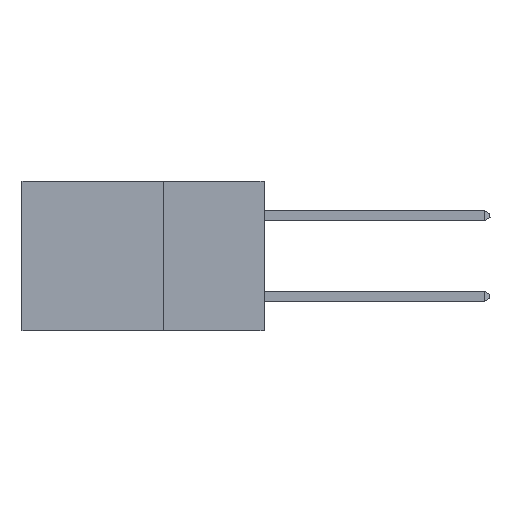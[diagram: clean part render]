
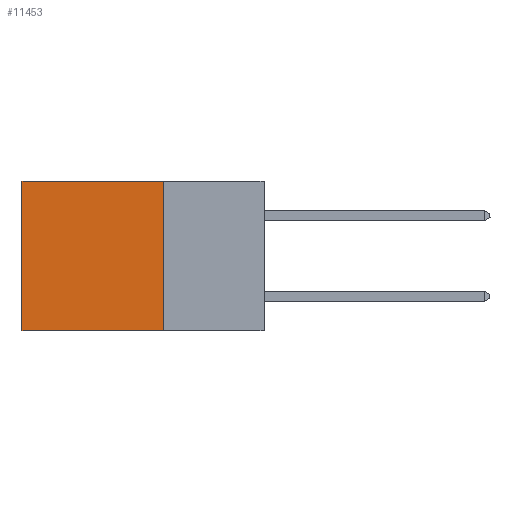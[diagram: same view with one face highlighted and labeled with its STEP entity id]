
A CAD part, left-side view. The second image highlights one B-rep face of the part: STEP entity #11453.
In plain terms, the highlighted planar face has unit normal (-1, 0, 0).
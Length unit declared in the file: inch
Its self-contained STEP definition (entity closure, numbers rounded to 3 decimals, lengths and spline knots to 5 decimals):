
#175 = AXIS2_PLACEMENT_3D ( 'NONE', #6943, #1509, #12089 ) ;
#1000 = ORIENTED_EDGE ( 'NONE', *, *, #13072, .F. ) ;
#1509 = DIRECTION ( 'NONE',  ( 1., 0., 0. ) ) ;
#1548 = EDGE_CURVE ( 'NONE', #6467, #7596, #8917, .T. ) ;
#3827 = CARTESIAN_POINT ( 'NONE',  ( 0.298, 0.6, -0.37 ) ) ;
#4586 = DIRECTION ( 'NONE',  ( 0., 0., -1. ) ) ;
#4882 = VECTOR ( 'NONE', #9130, 39.37008 ) ;
#6467 = VERTEX_POINT ( 'NONE', #10850 ) ;
#6473 = CARTESIAN_POINT ( 'NONE',  ( 0.298, 0.25, -0.37 ) ) ;
#6724 = LINE ( 'NONE', #9670, #13914 ) ;
#6943 = CARTESIAN_POINT ( 'NONE',  ( 0.298, 0.25, 0. ) ) ;
#7167 = VERTEX_POINT ( 'NONE', #3827 ) ;
#7596 = VERTEX_POINT ( 'NONE', #7931 ) ;
#7931 = CARTESIAN_POINT ( 'NONE',  ( 0.298, 0.6, 0. ) ) ;
#8087 = VECTOR ( 'NONE', #16560, 39.37008 ) ;
#8239 = PLANE ( 'NONE',  #175 ) ;
#8670 = DIRECTION ( 'NONE',  ( 0., 0., -1. ) ) ;
#8917 = LINE ( 'NONE', #13822, #8087 ) ;
#9020 = VERTEX_POINT ( 'NONE', #11935 ) ;
#9130 = DIRECTION ( 'NONE',  ( 0., 1., 0. ) ) ;
#9481 = LINE ( 'NONE', #15187, #11712 ) ;
#9642 = ORIENTED_EDGE ( 'NONE', *, *, #15500, .F. ) ;
#9670 = CARTESIAN_POINT ( 'NONE',  ( 0.298, 0.6, 0. ) ) ;
#9924 = FACE_OUTER_BOUND ( 'NONE', #10275, .T. ) ;
#10240 = ORIENTED_EDGE ( 'NONE', *, *, #1548, .T. ) ;
#10275 = EDGE_LOOP ( 'NONE', ( #15477, #9642, #1000, #10240 ) ) ;
#10850 = CARTESIAN_POINT ( 'NONE',  ( 0.298, 0.25, 0. ) ) ;
#11453 = ADVANCED_FACE ( 'NONE', ( #9924 ), #8239, .F. ) ;
#11712 = VECTOR ( 'NONE', #8670, 39.37008 ) ;
#11935 = CARTESIAN_POINT ( 'NONE',  ( 0.298, 0.25, -0.37 ) ) ;
#12089 = DIRECTION ( 'NONE',  ( 0., 0., -1. ) ) ;
#12241 = LINE ( 'NONE', #6473, #4882 ) ;
#13072 = EDGE_CURVE ( 'NONE', #6467, #9020, #9481, .T. ) ;
#13822 = CARTESIAN_POINT ( 'NONE',  ( 0.298, 0.25, 0. ) ) ;
#13914 = VECTOR ( 'NONE', #4586, 39.37008 ) ;
#14877 = EDGE_CURVE ( 'NONE', #7596, #7167, #6724, .T. ) ;
#15187 = CARTESIAN_POINT ( 'NONE',  ( 0.298, 0.25, 0. ) ) ;
#15477 = ORIENTED_EDGE ( 'NONE', *, *, #14877, .T. ) ;
#15500 = EDGE_CURVE ( 'NONE', #9020, #7167, #12241, .T. ) ;
#16560 = DIRECTION ( 'NONE',  ( 0., 1., 0. ) ) ;
